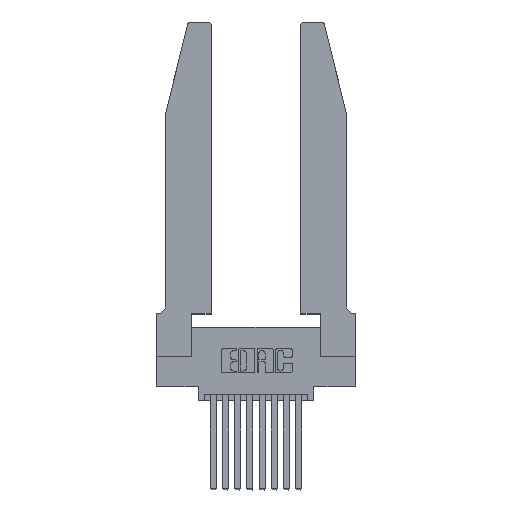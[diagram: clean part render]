
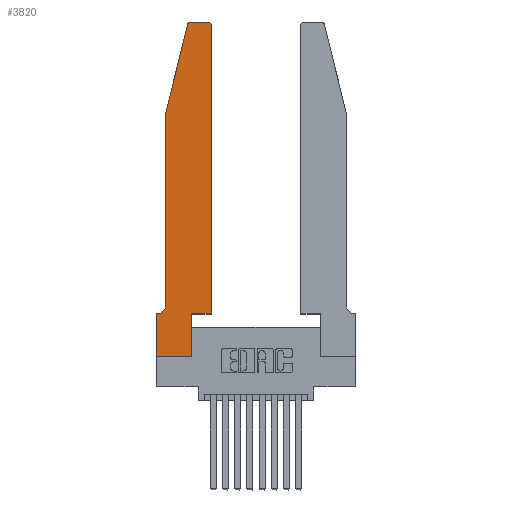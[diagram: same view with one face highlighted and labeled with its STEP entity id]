
A CAD part, top view. The second image highlights one B-rep face of the part: STEP entity #3820.
In plain terms, the highlighted planar face has unit normal (0, 0, 1).
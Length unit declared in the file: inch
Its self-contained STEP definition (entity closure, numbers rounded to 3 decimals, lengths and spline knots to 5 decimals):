
#5 = ORIENTED_EDGE ( 'NONE', *, *, #15232, .T. ) ;
#125 = CARTESIAN_POINT ( 'NONE',  ( 0.2605, 2.75, 0.37 ) ) ;
#235 = ORIENTED_EDGE ( 'NONE', *, *, #7940, .T. ) ;
#241 = LINE ( 'NONE', #4397, #12670 ) ;
#259 = EDGE_CURVE ( 'NONE', #6310, #4663, #3973, .T. ) ;
#377 = ORIENTED_EDGE ( 'NONE', *, *, #3826, .T. ) ;
#399 = AXIS2_PLACEMENT_3D ( 'NONE', #986, #9418, #2218 ) ;
#461 = ORIENTED_EDGE ( 'NONE', *, *, #5256, .T. ) ;
#604 = EDGE_CURVE ( 'NONE', #2801, #6310, #6247, .T. ) ;
#626 = LINE ( 'NONE', #13838, #3489 ) ;
#664 = CIRCLE ( 'NONE', #399, 0.03 ) ;
#696 = VERTEX_POINT ( 'NONE', #12197 ) ;
#733 = VECTOR ( 'NONE', #1217, 39.37008 ) ;
#817 = VERTEX_POINT ( 'NONE', #8159 ) ;
#822 = ORIENTED_EDGE ( 'NONE', *, *, #4889, .T. ) ;
#918 = DIRECTION ( 'NONE',  ( 0., 1., 0. ) ) ;
#940 = VERTEX_POINT ( 'NONE', #4407 ) ;
#959 = ORIENTED_EDGE ( 'NONE', *, *, #10004, .T. ) ;
#986 = CARTESIAN_POINT ( 'NONE',  ( 0.284, 2.72, 0.37 ) ) ;
#1112 = VERTEX_POINT ( 'NONE', #2386 ) ;
#1121 = ORIENTED_EDGE ( 'NONE', *, *, #10042, .T. ) ;
#1122 = VECTOR ( 'NONE', #3949, 39.37008 ) ;
#1217 = DIRECTION ( 'NONE',  ( 0., 1., 0. ) ) ;
#1230 = ORIENTED_EDGE ( 'NONE', *, *, #5039, .T. ) ;
#1354 = CARTESIAN_POINT ( 'NONE',  ( 0.4505, 0.35, 0.37 ) ) ;
#1428 = ORIENTED_EDGE ( 'NONE', *, *, #604, .T. ) ;
#1442 = VECTOR ( 'NONE', #10693, 39.37008 ) ;
#1988 = ORIENTED_EDGE ( 'NONE', *, *, #259, .T. ) ;
#2090 = ORIENTED_EDGE ( 'NONE', *, *, #11546, .T. ) ;
#2218 = DIRECTION ( 'NONE',  ( 1., 0., 0. ) ) ;
#2386 = CARTESIAN_POINT ( 'NONE',  ( 0., 0.35, 0.37 ) ) ;
#2705 = CARTESIAN_POINT ( 'NONE',  ( 0.0755, 2., 0.37 ) ) ;
#2801 = VERTEX_POINT ( 'NONE', #4114 ) ;
#2835 = VERTEX_POINT ( 'NONE', #5151 ) ;
#3003 = VECTOR ( 'NONE', #14461, 39.37008 ) ;
#3489 = VECTOR ( 'NONE', #12702, 39.37008 ) ;
#3516 = CARTESIAN_POINT ( 'NONE',  ( 0., 0.35, 0.37 ) ) ;
#3820 = ADVANCED_FACE ( 'NONE', ( #7484 ), #13097, .T. ) ;
#3826 = EDGE_CURVE ( 'NONE', #696, #2835, #10657, .T. ) ;
#3908 = CARTESIAN_POINT ( 'NONE',  ( 0.4505, 2.72, 0.37 ) ) ;
#3944 = DIRECTION ( 'NONE',  ( 0., 0., -1. ) ) ;
#3949 = DIRECTION ( 'NONE',  ( -0.239, -0.971, 0. ) ) ;
#3973 = LINE ( 'NONE', #1354, #733 ) ;
#4114 = CARTESIAN_POINT ( 'NONE',  ( 0.2865, 0.35, 0.37 ) ) ;
#4397 = CARTESIAN_POINT ( 'NONE',  ( 0., 0., 0.37 ) ) ;
#4407 = CARTESIAN_POINT ( 'NONE',  ( 0.4205, 2.75, 0.37 ) ) ;
#4663 = VERTEX_POINT ( 'NONE', #3908 ) ;
#4889 = EDGE_CURVE ( 'NONE', #817, #1112, #12684, .T. ) ;
#5039 = EDGE_CURVE ( 'NONE', #12296, #2801, #15108, .T. ) ;
#5151 = CARTESIAN_POINT ( 'NONE',  ( 0.0755, 0.42, 0.37 ) ) ;
#5256 = EDGE_CURVE ( 'NONE', #2835, #817, #14157, .T. ) ;
#6152 = CARTESIAN_POINT ( 'NONE',  ( 0.4205, 2.72, 0.37 ) ) ;
#6247 = LINE ( 'NONE', #15175, #3003 ) ;
#6310 = VERTEX_POINT ( 'NONE', #10338 ) ;
#7150 = DIRECTION ( 'NONE',  ( 1., 0., 0. ) ) ;
#7252 = VERTEX_POINT ( 'NONE', #14681 ) ;
#7262 = LINE ( 'NONE', #125, #10440 ) ;
#7322 = DIRECTION ( 'NONE',  ( 1., 0., 0. ) ) ;
#7385 = DIRECTION ( 'NONE',  ( -1., 0., 0. ) ) ;
#7484 = FACE_OUTER_BOUND ( 'NONE', #9232, .T. ) ;
#7940 = EDGE_CURVE ( 'NONE', #8565, #696, #13894, .T. ) ;
#7949 = CARTESIAN_POINT ( 'NONE',  ( 0.0755, 0.35, 0.37 ) ) ;
#8159 = CARTESIAN_POINT ( 'NONE',  ( 0.0055, 0.35, 0.37 ) ) ;
#8565 = VERTEX_POINT ( 'NONE', #9121 ) ;
#9121 = CARTESIAN_POINT ( 'NONE',  ( 0.25487, 2.72718, 0.37 ) ) ;
#9150 = DIRECTION ( 'NONE',  ( -1., 0., 0. ) ) ;
#9232 = EDGE_LOOP ( 'NONE', ( #14884, #5, #235, #377, #461, #822, #959, #1121, #1230, #1428, #1988, #2090 ) ) ;
#9347 = CARTESIAN_POINT ( 'NONE',  ( 0.2865, 0.35, 0.37 ) ) ;
#9418 = DIRECTION ( 'NONE',  ( 0., 0., 1. ) ) ;
#9450 = AXIS2_PLACEMENT_3D ( 'NONE', #6152, #14465, #7322 ) ;
#9513 = VECTOR ( 'NONE', #9150, 39.37008 ) ;
#9800 = EDGE_CURVE ( 'NONE', #940, #13934, #7262, .T. ) ;
#10004 = EDGE_CURVE ( 'NONE', #1112, #7252, #626, .T. ) ;
#10042 = EDGE_CURVE ( 'NONE', #7252, #12296, #241, .T. ) ;
#10273 = CARTESIAN_POINT ( 'NONE',  ( 0.284, 2.75, 0.37 ) ) ;
#10338 = CARTESIAN_POINT ( 'NONE',  ( 0.4505, 0.35, 0.37 ) ) ;
#10440 = VECTOR ( 'NONE', #7385, 39.37008 ) ;
#10657 = LINE ( 'NONE', #15486, #1442 ) ;
#10693 = DIRECTION ( 'NONE',  ( 0., -1., 0. ) ) ;
#11113 = CARTESIAN_POINT ( 'NONE',  ( 0.0055, 0.42, 0.37 ) ) ;
#11546 = EDGE_CURVE ( 'NONE', #4663, #940, #15421, .T. ) ;
#11551 = DIRECTION ( 'NONE',  ( 1., 0., 0. ) ) ;
#12197 = CARTESIAN_POINT ( 'NONE',  ( 0.0755, 2., 0.37 ) ) ;
#12296 = VERTEX_POINT ( 'NONE', #13932 ) ;
#12326 = DIRECTION ( 'NONE',  ( -1., 0., 0. ) ) ;
#12349 = AXIS2_PLACEMENT_3D ( 'NONE', #11113, #3944, #12326 ) ;
#12670 = VECTOR ( 'NONE', #11551, 39.37008 ) ;
#12684 = LINE ( 'NONE', #7949, #9513 ) ;
#12702 = DIRECTION ( 'NONE',  ( 0., -1., 0. ) ) ;
#13097 = PLANE ( 'NONE',  #14323 ) ;
#13600 = VECTOR ( 'NONE', #918, 39.37008 ) ;
#13838 = CARTESIAN_POINT ( 'NONE',  ( 0., 0., 0.37 ) ) ;
#13894 = LINE ( 'NONE', #2705, #1122 ) ;
#13932 = CARTESIAN_POINT ( 'NONE',  ( 0.2865, 0., 0.37 ) ) ;
#13934 = VERTEX_POINT ( 'NONE', #10273 ) ;
#14157 = CIRCLE ( 'NONE', #12349, 0.07 ) ;
#14287 = DIRECTION ( 'NONE',  ( 0., 0., 1. ) ) ;
#14323 = AXIS2_PLACEMENT_3D ( 'NONE', #3516, #14287, #7150 ) ;
#14461 = DIRECTION ( 'NONE',  ( 1., 0., 0. ) ) ;
#14465 = DIRECTION ( 'NONE',  ( 0., 0., 1. ) ) ;
#14681 = CARTESIAN_POINT ( 'NONE',  ( 0., 0., 0.37 ) ) ;
#14884 = ORIENTED_EDGE ( 'NONE', *, *, #9800, .T. ) ;
#15108 = LINE ( 'NONE', #9347, #13600 ) ;
#15175 = CARTESIAN_POINT ( 'NONE',  ( 0.4505, 0.35, 0.37 ) ) ;
#15232 = EDGE_CURVE ( 'NONE', #13934, #8565, #664, .T. ) ;
#15421 = CIRCLE ( 'NONE', #9450, 0.03 ) ;
#15486 = CARTESIAN_POINT ( 'NONE',  ( 0.0755, 2., 0.37 ) ) ;
